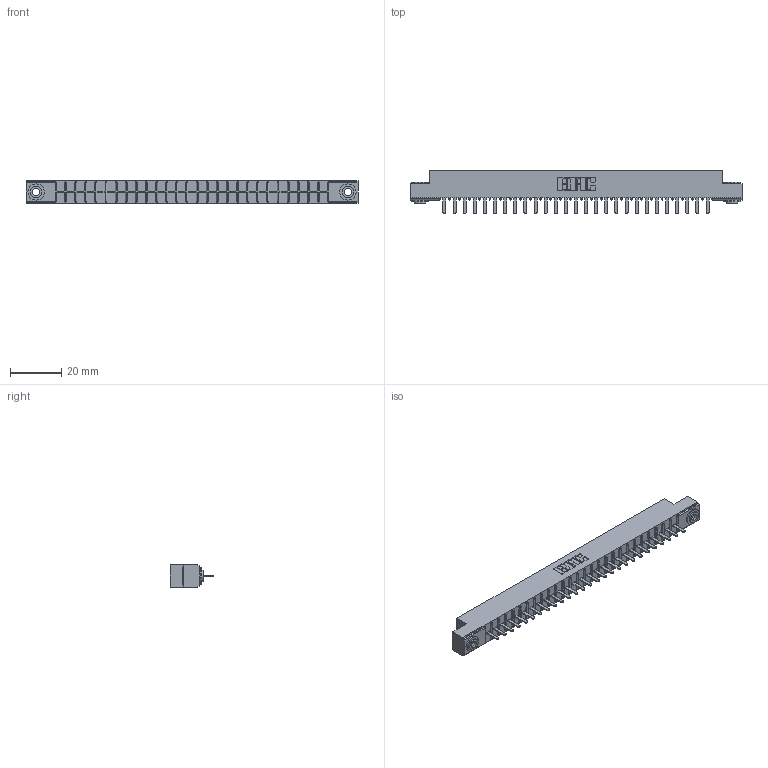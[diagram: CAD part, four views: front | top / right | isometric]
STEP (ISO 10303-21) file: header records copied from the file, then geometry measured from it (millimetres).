
FILE_DESCRIPTION (( 'STEP AP203' ), '1' );
FILE_NAME ('316-027-420-103.STEP', '2020-09-22T22:56:09', ( '' ), ( '' ), 'SwSTEP 2.0', 'SolidWorks 2020', '' );
FILE_SCHEMA (( 'CONFIG_CONTROL_DESIGN' ));
Length unit declared in the file: inch
Products named in the file (4): 345-250-002_345-250-002-102; 316-027-420-103; 306-290-001_120; 306 Part_.156 Dia
Assembly tree (30 placements, depth 2):
  316-027-420-103
    306 Part_.156 Dia
    306-290-001_120  x27
    345-250-002_345-250-002-102  x2
Bounding box: 130 x 17.12 x 8.71 mm (x, y, z)
Volume: 8922 mm3; surface area: 13595.2 mm2
Topology: 30 solids, 30 shells, 2058 faces, 5747 edges, 3682 vertices
Faces by surface type: plane 1361, cylinder 581, sphere 108, cone 8
Entity records: 28143 total; most frequent: CARTESIAN_POINT 4701, DIRECTION 4651, ORIENTED_EDGE 4650, EDGE_CURVE 2325, LINE 1803, VECTOR 1803, VERTEX_POINT 1474, AXIS2_PLACEMENT_3D 1424
